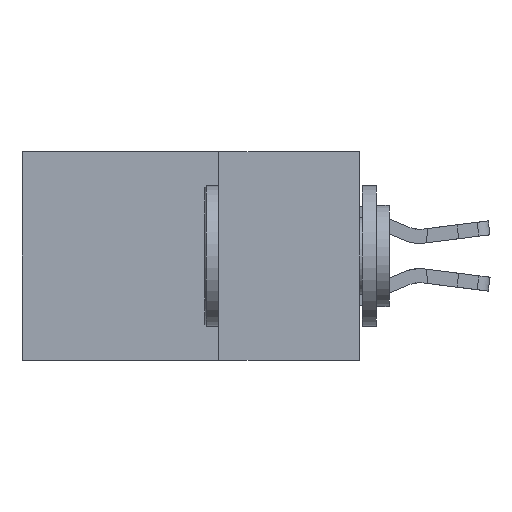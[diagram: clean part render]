
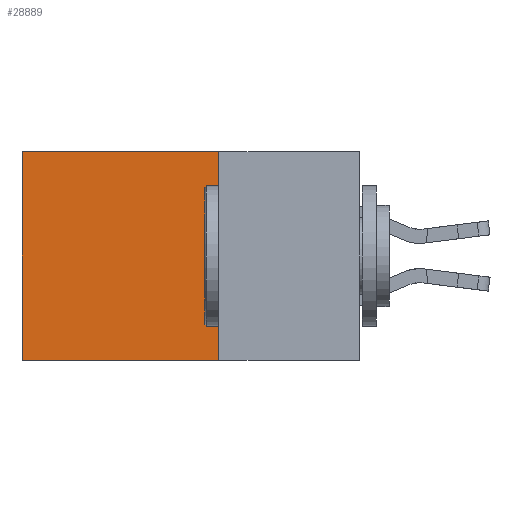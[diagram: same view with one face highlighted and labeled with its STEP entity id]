
A CAD part, left-side view. The second image highlights one B-rep face of the part: STEP entity #28889.
In plain terms, the highlighted planar face has unit normal (-1, 0, 0).
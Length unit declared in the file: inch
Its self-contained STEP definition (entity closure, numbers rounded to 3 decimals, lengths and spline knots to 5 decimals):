
#1154 = CARTESIAN_POINT ( 'NONE',  ( 0.2875, 0.25, 0. ) ) ;
#1367 = DIRECTION ( 'NONE',  ( 0., 0., -1. ) ) ;
#1675 = EDGE_CURVE ( 'NONE', #20252, #20928, #14844, .T. ) ;
#3716 = DIRECTION ( 'NONE',  ( 1., 0., 0. ) ) ;
#4268 = VECTOR ( 'NONE', #17758, 39.37008 ) ;
#5311 = CARTESIAN_POINT ( 'NONE',  ( 0.2875, 0.25, -0.37 ) ) ;
#7109 = FACE_OUTER_BOUND ( 'NONE', #29557, .T. ) ;
#7495 = LINE ( 'NONE', #9246, #24772 ) ;
#7646 = CARTESIAN_POINT ( 'NONE',  ( 0.2875, 0.25, 0. ) ) ;
#7935 = ORIENTED_EDGE ( 'NONE', *, *, #13567, .F. ) ;
#9246 = CARTESIAN_POINT ( 'NONE',  ( 0.2875, 0.6, 0. ) ) ;
#9845 = VERTEX_POINT ( 'NONE', #31509 ) ;
#10349 = ORIENTED_EDGE ( 'NONE', *, *, #23293, .F. ) ;
#11779 = EDGE_CURVE ( 'NONE', #20928, #9845, #7495, .T. ) ;
#12376 = ORIENTED_EDGE ( 'NONE', *, *, #11779, .T. ) ;
#13567 = EDGE_CURVE ( 'NONE', #20252, #22784, #29636, .T. ) ;
#14844 = LINE ( 'NONE', #27218, #15360 ) ;
#15360 = VECTOR ( 'NONE', #29777, 39.37008 ) ;
#17219 = DIRECTION ( 'NONE',  ( 0., 0., -1. ) ) ;
#17758 = DIRECTION ( 'NONE',  ( 0., 1., 0. ) ) ;
#18720 = VECTOR ( 'NONE', #17219, 39.37008 ) ;
#19210 = CARTESIAN_POINT ( 'NONE',  ( 0.2875, 0.6, 0. ) ) ;
#19214 = DIRECTION ( 'NONE',  ( 0., 0., -1. ) ) ;
#20252 = VERTEX_POINT ( 'NONE', #7646 ) ;
#20714 = LINE ( 'NONE', #30812, #4268 ) ;
#20928 = VERTEX_POINT ( 'NONE', #19210 ) ;
#22784 = VERTEX_POINT ( 'NONE', #5311 ) ;
#23293 = EDGE_CURVE ( 'NONE', #22784, #9845, #20714, .T. ) ;
#24733 = AXIS2_PLACEMENT_3D ( 'NONE', #1154, #3716, #19214 ) ;
#24772 = VECTOR ( 'NONE', #1367, 39.37008 ) ;
#27218 = CARTESIAN_POINT ( 'NONE',  ( 0.2875, 0.25, 0. ) ) ;
#28889 = ADVANCED_FACE ( 'NONE', ( #7109 ), #32415, .F. ) ;
#29557 = EDGE_LOOP ( 'NONE', ( #12376, #10349, #7935, #29915 ) ) ;
#29636 = LINE ( 'NONE', #29845, #18720 ) ;
#29777 = DIRECTION ( 'NONE',  ( 0., 1., 0. ) ) ;
#29845 = CARTESIAN_POINT ( 'NONE',  ( 0.2875, 0.25, 0. ) ) ;
#29915 = ORIENTED_EDGE ( 'NONE', *, *, #1675, .T. ) ;
#30812 = CARTESIAN_POINT ( 'NONE',  ( 0.2875, 0.25, -0.37 ) ) ;
#31509 = CARTESIAN_POINT ( 'NONE',  ( 0.2875, 0.6, -0.37 ) ) ;
#32415 = PLANE ( 'NONE',  #24733 ) ;
